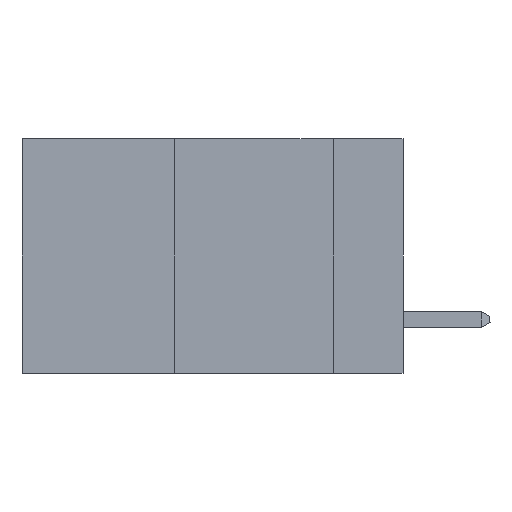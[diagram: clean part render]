
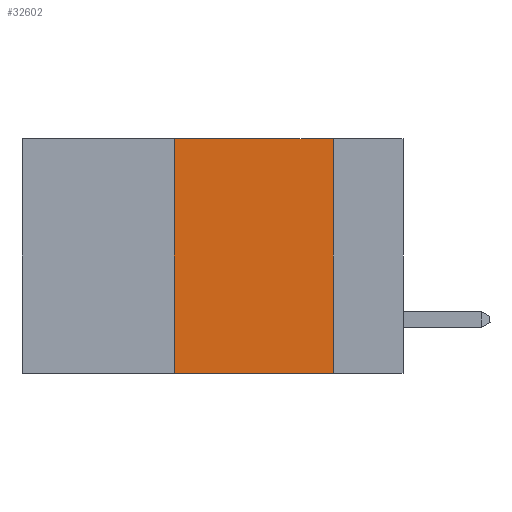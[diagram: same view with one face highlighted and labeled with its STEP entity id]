
A CAD part, left-side view. The second image highlights one B-rep face of the part: STEP entity #32602.
In plain terms, the highlighted planar face has unit normal (-1, 0, 0).
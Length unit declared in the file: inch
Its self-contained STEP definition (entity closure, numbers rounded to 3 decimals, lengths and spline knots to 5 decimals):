
#888 = VECTOR ( 'NONE', #1493, 39.37008 ) ;
#1493 = DIRECTION ( 'NONE',  ( 0., 0., 1. ) ) ;
#5716 = EDGE_CURVE ( 'NONE', #25762, #24685, #25110, .T. ) ;
#6492 = VERTEX_POINT ( 'NONE', #25065 ) ;
#7061 = ORIENTED_EDGE ( 'NONE', *, *, #5716, .T. ) ;
#7116 = DIRECTION ( 'NONE',  ( 0., 0., -1. ) ) ;
#9758 = CARTESIAN_POINT ( 'NONE',  ( 0., 0.11, 0. ) ) ;
#10124 = DIRECTION ( 'NONE',  ( 0., -1., 0. ) ) ;
#10711 = VERTEX_POINT ( 'NONE', #42061 ) ;
#11096 = PLANE ( 'NONE',  #42990 ) ;
#15930 = LINE ( 'NONE', #9758, #21433 ) ;
#16351 = ORIENTED_EDGE ( 'NONE', *, *, #21138, .F. ) ;
#18860 = CARTESIAN_POINT ( 'NONE',  ( 0., 0.36, 0. ) ) ;
#19063 = VECTOR ( 'NONE', #31119, 39.37008 ) ;
#19386 = FACE_OUTER_BOUND ( 'NONE', #21365, .T. ) ;
#20991 = DIRECTION ( 'NONE',  ( 0., 0., -1. ) ) ;
#21138 = EDGE_CURVE ( 'NONE', #10711, #6492, #40598, .T. ) ;
#21247 = EDGE_CURVE ( 'NONE', #6492, #24685, #15930, .T. ) ;
#21365 = EDGE_LOOP ( 'NONE', ( #40212, #16351, #30873, #7061 ) ) ;
#21433 = VECTOR ( 'NONE', #20991, 39.37008 ) ;
#21692 = CARTESIAN_POINT ( 'NONE',  ( 0., 0.6, 0. ) ) ;
#24585 = LINE ( 'NONE', #18860, #888 ) ;
#24685 = VERTEX_POINT ( 'NONE', #36646 ) ;
#25065 = CARTESIAN_POINT ( 'NONE',  ( 0., 0.11, 0. ) ) ;
#25110 = LINE ( 'NONE', #34352, #19063 ) ;
#25399 = EDGE_CURVE ( 'NONE', #25762, #10711, #24585, .T. ) ;
#25762 = VERTEX_POINT ( 'NONE', #26817 ) ;
#26817 = CARTESIAN_POINT ( 'NONE',  ( 0., 0.36, -0.37 ) ) ;
#27627 = CARTESIAN_POINT ( 'NONE',  ( 0., 0.6, 0. ) ) ;
#30873 = ORIENTED_EDGE ( 'NONE', *, *, #25399, .F. ) ;
#31119 = DIRECTION ( 'NONE',  ( 0., -1., 0. ) ) ;
#32602 = ADVANCED_FACE ( 'NONE', ( #19386 ), #11096, .F. ) ;
#34352 = CARTESIAN_POINT ( 'NONE',  ( 0., 0.6, -0.37 ) ) ;
#36646 = CARTESIAN_POINT ( 'NONE',  ( 0., 0.11, -0.37 ) ) ;
#38589 = DIRECTION ( 'NONE',  ( 1., 0., 0. ) ) ;
#40212 = ORIENTED_EDGE ( 'NONE', *, *, #21247, .F. ) ;
#40598 = LINE ( 'NONE', #27627, #45008 ) ;
#42061 = CARTESIAN_POINT ( 'NONE',  ( 0., 0.36, 0. ) ) ;
#42990 = AXIS2_PLACEMENT_3D ( 'NONE', #21692, #38589, #7116 ) ;
#45008 = VECTOR ( 'NONE', #10124, 39.37008 ) ;
